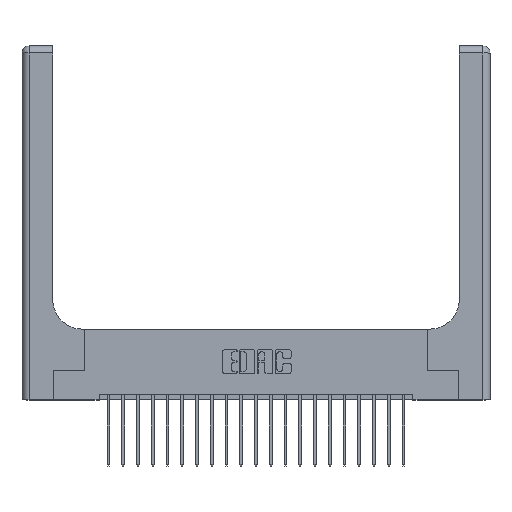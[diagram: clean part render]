
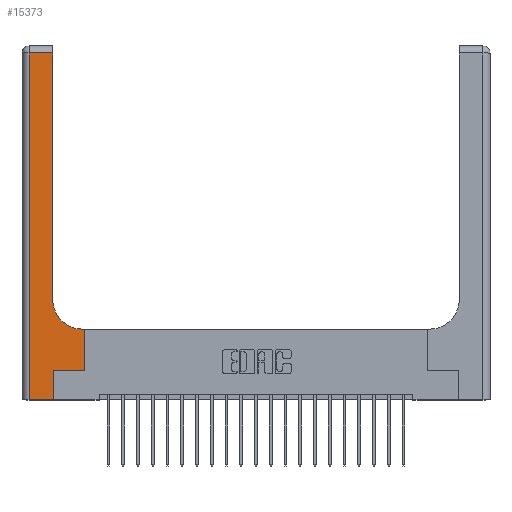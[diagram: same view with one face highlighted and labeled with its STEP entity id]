
A CAD part, top view. The second image highlights one B-rep face of the part: STEP entity #15373.
In plain terms, the highlighted planar face has unit normal (0, 0, 1).
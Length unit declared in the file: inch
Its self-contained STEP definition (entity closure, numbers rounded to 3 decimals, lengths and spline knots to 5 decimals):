
#677 = CARTESIAN_POINT ( 'NONE',  ( 0.51, 0.85, 0.37 ) ) ;
#901 = EDGE_CURVE ( 'NONE', #1060, #6737, #17729, .T. ) ;
#1060 = VERTEX_POINT ( 'NONE', #1246 ) ;
#1233 = EDGE_CURVE ( 'NONE', #18478, #1060, #17041, .T. ) ;
#1246 = CARTESIAN_POINT ( 'NONE',  ( 0.528, 0.6, 0.37 ) ) ;
#1886 = CARTESIAN_POINT ( 'NONE',  ( 0.528, 0.25, 0.37 ) ) ;
#2503 = VECTOR ( 'NONE', #8747, 39.37008 ) ;
#2631 = ORIENTED_EDGE ( 'NONE', *, *, #901, .T. ) ;
#2666 = CARTESIAN_POINT ( 'NONE',  ( 0.06, 2.94, 0.37 ) ) ;
#2850 = CARTESIAN_POINT ( 'NONE',  ( 0.265, 0.25, 0.37 ) ) ;
#2919 = EDGE_CURVE ( 'NONE', #9081, #3374, #12530, .T. ) ;
#2923 = DIRECTION ( 'NONE',  ( -1., 0., 0. ) ) ;
#2968 = LINE ( 'NONE', #9804, #5329 ) ;
#3374 = VERTEX_POINT ( 'NONE', #13796 ) ;
#3817 = VECTOR ( 'NONE', #5159, 39.37008 ) ;
#3882 = VERTEX_POINT ( 'NONE', #9249 ) ;
#3963 = EDGE_LOOP ( 'NONE', ( #18438, #8908, #16325, #7764, #11831, #16680, #19219, #2631, #22014 ) ) ;
#4238 = DIRECTION ( 'NONE',  ( 0., 1., 0. ) ) ;
#4331 = EDGE_CURVE ( 'NONE', #6737, #3882, #16782, .T. ) ;
#4390 = PLANE ( 'NONE',  #15372 ) ;
#4767 = DIRECTION ( 'NONE',  ( 0., -1., 0. ) ) ;
#5159 = DIRECTION ( 'NONE',  ( 1., 0., 0. ) ) ;
#5186 = VECTOR ( 'NONE', #19860, 39.37008 ) ;
#5298 = VERTEX_POINT ( 'NONE', #2666 ) ;
#5305 = LINE ( 'NONE', #20437, #18369 ) ;
#5329 = VECTOR ( 'NONE', #4767, 39.37008 ) ;
#5716 = CARTESIAN_POINT ( 'NONE',  ( 0.06, 0., 0.37 ) ) ;
#5874 = DIRECTION ( 'NONE',  ( 0., 0., -1. ) ) ;
#6035 = EDGE_CURVE ( 'NONE', #10635, #9081, #17248, .T. ) ;
#6737 = VERTEX_POINT ( 'NONE', #12734 ) ;
#7097 = DIRECTION ( 'NONE',  ( 0., 1., 0. ) ) ;
#7132 = AXIS2_PLACEMENT_3D ( 'NONE', #677, #5874, #20998 ) ;
#7497 = VECTOR ( 'NONE', #21565, 39.37008 ) ;
#7764 = ORIENTED_EDGE ( 'NONE', *, *, #6035, .T. ) ;
#7864 = CARTESIAN_POINT ( 'NONE',  ( 0.26, 0.6, 0.37 ) ) ;
#8747 = DIRECTION ( 'NONE',  ( 0., 1., 0. ) ) ;
#8908 = ORIENTED_EDGE ( 'NONE', *, *, #17469, .T. ) ;
#9081 = VERTEX_POINT ( 'NONE', #12681 ) ;
#9170 = CARTESIAN_POINT ( 'NONE',  ( 0.265, 0., 0.37 ) ) ;
#9249 = CARTESIAN_POINT ( 'NONE',  ( 0.26, 0.85, 0.37 ) ) ;
#9710 = DIRECTION ( 'NONE',  ( -1., 0., 0. ) ) ;
#9758 = CARTESIAN_POINT ( 'NONE',  ( 0., 3., 0.37 ) ) ;
#9804 = CARTESIAN_POINT ( 'NONE',  ( 0.06, 3., 0.37 ) ) ;
#10524 = CARTESIAN_POINT ( 'NONE',  ( 0., 0., 0.37 ) ) ;
#10635 = VERTEX_POINT ( 'NONE', #5716 ) ;
#11260 = LINE ( 'NONE', #2850, #7497 ) ;
#11831 = ORIENTED_EDGE ( 'NONE', *, *, #2919, .T. ) ;
#11872 = CARTESIAN_POINT ( 'NONE',  ( 0.26, 2.94, 0.37 ) ) ;
#12530 = LINE ( 'NONE', #9170, #14888 ) ;
#12681 = CARTESIAN_POINT ( 'NONE',  ( 0.265, 0., 0.37 ) ) ;
#12734 = CARTESIAN_POINT ( 'NONE',  ( 0.51, 0.6, 0.37 ) ) ;
#13082 = EDGE_CURVE ( 'NONE', #3374, #18478, #11260, .T. ) ;
#13180 = CARTESIAN_POINT ( 'NONE',  ( 0., 2.94, 0.37 ) ) ;
#13796 = CARTESIAN_POINT ( 'NONE',  ( 0.265, 0.25, 0.37 ) ) ;
#14442 = EDGE_CURVE ( 'NONE', #5298, #10635, #2968, .T. ) ;
#14888 = VECTOR ( 'NONE', #4238, 39.37008 ) ;
#15372 = AXIS2_PLACEMENT_3D ( 'NONE', #9758, #18278, #2923 ) ;
#15373 = ADVANCED_FACE ( 'NONE', ( #18504 ), #4390, .F. ) ;
#16325 = ORIENTED_EDGE ( 'NONE', *, *, #14442, .T. ) ;
#16537 = LINE ( 'NONE', #13180, #20818 ) ;
#16680 = ORIENTED_EDGE ( 'NONE', *, *, #13082, .T. ) ;
#16782 = CIRCLE ( 'NONE', #7132, 0.25 ) ;
#17041 = LINE ( 'NONE', #18725, #2503 ) ;
#17248 = LINE ( 'NONE', #10524, #3817 ) ;
#17469 = EDGE_CURVE ( 'NONE', #21401, #5298, #16537, .T. ) ;
#17729 = LINE ( 'NONE', #7864, #5186 ) ;
#18278 = DIRECTION ( 'NONE',  ( 0., 0., -1. ) ) ;
#18369 = VECTOR ( 'NONE', #7097, 39.37008 ) ;
#18438 = ORIENTED_EDGE ( 'NONE', *, *, #19175, .T. ) ;
#18478 = VERTEX_POINT ( 'NONE', #1886 ) ;
#18504 = FACE_OUTER_BOUND ( 'NONE', #3963, .T. ) ;
#18725 = CARTESIAN_POINT ( 'NONE',  ( 0.528, 0.25, 0.37 ) ) ;
#19175 = EDGE_CURVE ( 'NONE', #3882, #21401, #5305, .T. ) ;
#19219 = ORIENTED_EDGE ( 'NONE', *, *, #1233, .T. ) ;
#19860 = DIRECTION ( 'NONE',  ( -1., 0., 0. ) ) ;
#20437 = CARTESIAN_POINT ( 'NONE',  ( 0.26, 3., 0.37 ) ) ;
#20818 = VECTOR ( 'NONE', #9710, 39.37008 ) ;
#20998 = DIRECTION ( 'NONE',  ( 1., 0., 0. ) ) ;
#21401 = VERTEX_POINT ( 'NONE', #11872 ) ;
#21565 = DIRECTION ( 'NONE',  ( 1., 0., 0. ) ) ;
#22014 = ORIENTED_EDGE ( 'NONE', *, *, #4331, .T. ) ;
